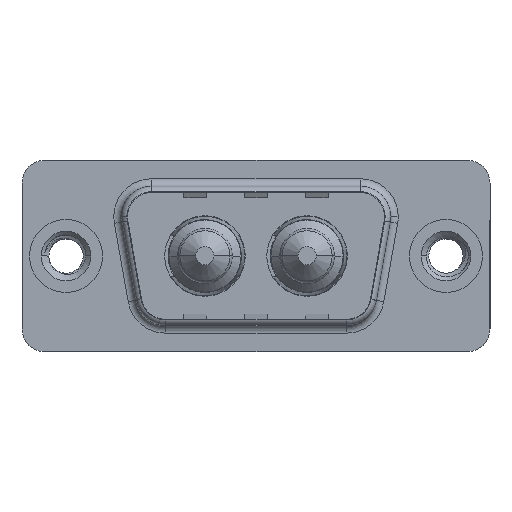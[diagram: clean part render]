
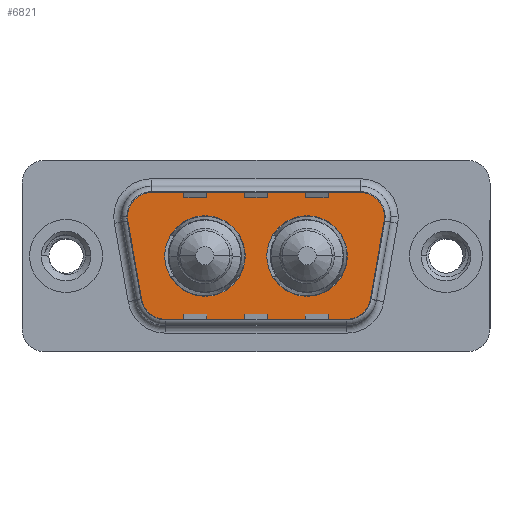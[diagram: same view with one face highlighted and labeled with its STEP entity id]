
A CAD part, top view. The second image highlights one B-rep face of the part: STEP entity #6821.
In plain terms, the highlighted planar face has unit normal (0, 0, 1).
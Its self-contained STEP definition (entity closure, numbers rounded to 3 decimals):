
#55 = DIRECTION ( 'NONE',  ( 1., 0., 0. ) ) ;
#293 = EDGE_CURVE ( 'NONE', #538, #6343, #3353, .T. ) ;
#428 = CARTESIAN_POINT ( 'NONE',  ( 5.436, 4.9, 0. ) ) ;
#538 = VERTEX_POINT ( 'NONE', #7679 ) ;
#563 = CARTESIAN_POINT ( 'NONE',  ( 19.564, 2.9, 0. ) ) ;
#599 = DIRECTION ( 'NONE',  ( 0., 0., 1. ) ) ;
#717 = CARTESIAN_POINT ( 'NONE',  ( 3.466, 2.553, 0. ) ) ;
#746 = AXIS2_PLACEMENT_3D ( 'NONE', #1592, #10124, #2827 ) ;
#830 = CARTESIAN_POINT ( 'NONE',  ( 6.49, 0., 0. ) ) ;
#866 = CARTESIAN_POINT ( 'NONE',  ( 21.534, 2.553, 0. ) ) ;
#883 = CIRCLE ( 'NONE', #5592, 2. ) ;
#1329 = AXIS2_PLACEMENT_3D ( 'NONE', #5317, #13799, #6526 ) ;
#1493 = VECTOR ( 'NONE', #1997, 1000. ) ;
#1539 = VERTEX_POINT ( 'NONE', #830 ) ;
#1551 = VERTEX_POINT ( 'NONE', #10765 ) ;
#1585 = CARTESIAN_POINT ( 'NONE',  ( 6.459, -4.9, 0. ) ) ;
#1592 = CARTESIAN_POINT ( 'NONE',  ( 15.86, 0., 0. ) ) ;
#1773 = DIRECTION ( 'NONE',  ( -1., 0., 0. ) ) ;
#1788 = DIRECTION ( 'NONE',  ( 1., 0., 0. ) ) ;
#1823 = CIRCLE ( 'NONE', #6727, 2. ) ;
#1856 = VERTEX_POINT ( 'NONE', #9873 ) ;
#1989 = DIRECTION ( 'NONE',  ( 0.174, -0.985, 0. ) ) ;
#1997 = DIRECTION ( 'NONE',  ( 0.174, 0.985, 0. ) ) ;
#2703 = DIRECTION ( 'NONE',  ( 0., 0., 1. ) ) ;
#2827 = DIRECTION ( 'NONE',  ( 1., 0., 0. ) ) ;
#2969 = VECTOR ( 'NONE', #1989, 1000. ) ;
#3025 = FACE_OUTER_BOUND ( 'NONE', #11076, .T. ) ;
#3049 = CIRCLE ( 'NONE', #9756, 2. ) ;
#3152 = CIRCLE ( 'NONE', #746, 2.65 ) ;
#3353 = LINE ( 'NONE', #4922, #12299 ) ;
#3422 = EDGE_CURVE ( 'NONE', #1551, #7633, #13109, .T. ) ;
#3642 = EDGE_LOOP ( 'NONE', ( #8192, #15733 ) ) ;
#3718 = CARTESIAN_POINT ( 'NONE',  ( 4.489, -3.247, 0. ) ) ;
#3866 = DIRECTION ( 'NONE',  ( 1., 0., 0. ) ) ;
#4012 = DIRECTION ( 'NONE',  ( 1., 0., 0. ) ) ;
#4110 = CARTESIAN_POINT ( 'NONE',  ( 19.564, 2.9, 0. ) ) ;
#4141 = VERTEX_POINT ( 'NONE', #13921 ) ;
#4147 = DIRECTION ( 'NONE',  ( -1., 0., 0. ) ) ;
#4219 = PLANE ( 'NONE',  #15092 ) ;
#4314 = EDGE_CURVE ( 'NONE', #1856, #4745, #14405, .T. ) ;
#4329 = VECTOR ( 'NONE', #7620, 1000. ) ;
#4400 = DIRECTION ( 'NONE',  ( 1., 0., 0. ) ) ;
#4431 = ORIENTED_EDGE ( 'NONE', *, *, #9809, .T. ) ;
#4470 = CARTESIAN_POINT ( 'NONE',  ( 21.534, 2.553, 0. ) ) ;
#4663 = DIRECTION ( 'NONE',  ( 0., 0., 1. ) ) ;
#4745 = VERTEX_POINT ( 'NONE', #866 ) ;
#4808 = VERTEX_POINT ( 'NONE', #3718 ) ;
#4902 = CIRCLE ( 'NONE', #13381, 2.65 ) ;
#4922 = CARTESIAN_POINT ( 'NONE',  ( 5.436, 4.9, 0. ) ) ;
#5101 = EDGE_CURVE ( 'NONE', #1539, #8948, #8860, .T. ) ;
#5166 = EDGE_CURVE ( 'NONE', #8948, #1539, #4902, .T. ) ;
#5316 = DIRECTION ( 'NONE',  ( -1., 0., 0. ) ) ;
#5317 = CARTESIAN_POINT ( 'NONE',  ( 6.459, -2.9, 0. ) ) ;
#5384 = AXIS2_PLACEMENT_3D ( 'NONE', #563, #9035, #1773 ) ;
#5399 = CARTESIAN_POINT ( 'NONE',  ( 18.541, -2.9, 0. ) ) ;
#5592 = AXIS2_PLACEMENT_3D ( 'NONE', #4110, #12606, #5316 ) ;
#5746 = VERTEX_POINT ( 'NONE', #7340 ) ;
#6104 = EDGE_CURVE ( 'NONE', #6343, #12043, #1823, .T. ) ;
#6165 = EDGE_LOOP ( 'NONE', ( #12387, #10317 ) ) ;
#6197 = LINE ( 'NONE', #717, #2969 ) ;
#6218 = CIRCLE ( 'NONE', #5384, 2. ) ;
#6321 = EDGE_CURVE ( 'NONE', #7633, #1551, #3152, .T. ) ;
#6343 = VERTEX_POINT ( 'NONE', #428 ) ;
#6526 = DIRECTION ( 'NONE',  ( -1., 0., 0. ) ) ;
#6613 = FACE_BOUND ( 'NONE', #3642, .T. ) ;
#6727 = AXIS2_PLACEMENT_3D ( 'NONE', #14624, #7315, #55 ) ;
#6821 = ADVANCED_FACE ( 'NONE', ( #13093, #6613, #3025 ), #4219, .T. ) ;
#6941 = CARTESIAN_POINT ( 'NONE',  ( 13.21, 0., 0. ) ) ;
#7241 = ORIENTED_EDGE ( 'NONE', *, *, #13550, .T. ) ;
#7315 = DIRECTION ( 'NONE',  ( 0., 0., 1. ) ) ;
#7340 = CARTESIAN_POINT ( 'NONE',  ( 18.541, -4.9, 0. ) ) ;
#7429 = CARTESIAN_POINT ( 'NONE',  ( 15.86, 0., 0. ) ) ;
#7620 = DIRECTION ( 'NONE',  ( 1., 0., 0. ) ) ;
#7633 = VERTEX_POINT ( 'NONE', #6941 ) ;
#7679 = CARTESIAN_POINT ( 'NONE',  ( 19.564, 4.9, 0. ) ) ;
#8192 = ORIENTED_EDGE ( 'NONE', *, *, #5166, .F. ) ;
#8565 = ORIENTED_EDGE ( 'NONE', *, *, #8621, .T. ) ;
#8621 = EDGE_CURVE ( 'NONE', #12043, #4808, #6197, .T. ) ;
#8741 = CARTESIAN_POINT ( 'NONE',  ( 9.14, 0., 0. ) ) ;
#8748 = AXIS2_PLACEMENT_3D ( 'NONE', #7429, #4663, #3866 ) ;
#8860 = CIRCLE ( 'NONE', #10159, 2.65 ) ;
#8948 = VERTEX_POINT ( 'NONE', #9760 ) ;
#9035 = DIRECTION ( 'NONE',  ( 0., 0., 1. ) ) ;
#9057 = DIRECTION ( 'NONE',  ( 0., 0., 1. ) ) ;
#9194 = EDGE_CURVE ( 'NONE', #4808, #14980, #14551, .T. ) ;
#9359 = ORIENTED_EDGE ( 'NONE', *, *, #12990, .T. ) ;
#9556 = ORIENTED_EDGE ( 'NONE', *, *, #293, .T. ) ;
#9738 = ORIENTED_EDGE ( 'NONE', *, *, #9194, .T. ) ;
#9756 = AXIS2_PLACEMENT_3D ( 'NONE', #9983, #2703, #11215 ) ;
#9760 = CARTESIAN_POINT ( 'NONE',  ( 11.79, 0., 0. ) ) ;
#9809 = EDGE_CURVE ( 'NONE', #14980, #5746, #13982, .T. ) ;
#9873 = CARTESIAN_POINT ( 'NONE',  ( 20.511, -3.247, 0. ) ) ;
#9983 = CARTESIAN_POINT ( 'NONE',  ( 18.541, -2.9, 0. ) ) ;
#10124 = DIRECTION ( 'NONE',  ( 0., 0., 1. ) ) ;
#10159 = AXIS2_PLACEMENT_3D ( 'NONE', #15430, #13688, #4012 ) ;
#10317 = ORIENTED_EDGE ( 'NONE', *, *, #6321, .F. ) ;
#10421 = ORIENTED_EDGE ( 'NONE', *, *, #11082, .T. ) ;
#10713 = ORIENTED_EDGE ( 'NONE', *, *, #6104, .T. ) ;
#10755 = CARTESIAN_POINT ( 'NONE',  ( 3.466, 2.553, 0. ) ) ;
#10765 = CARTESIAN_POINT ( 'NONE',  ( 18.51, 0., 0. ) ) ;
#11076 = EDGE_LOOP ( 'NONE', ( #10421, #11762, #9359, #7241, #9556, #10713, #8565, #9738, #4431 ) ) ;
#11082 = EDGE_CURVE ( 'NONE', #5746, #1856, #3049, .T. ) ;
#11215 = DIRECTION ( 'NONE',  ( 1., 0., 0. ) ) ;
#11762 = ORIENTED_EDGE ( 'NONE', *, *, #4314, .T. ) ;
#12043 = VERTEX_POINT ( 'NONE', #10755 ) ;
#12299 = VECTOR ( 'NONE', #4147, 1000. ) ;
#12387 = ORIENTED_EDGE ( 'NONE', *, *, #3422, .F. ) ;
#12606 = DIRECTION ( 'NONE',  ( 0., 0., 1. ) ) ;
#12990 = EDGE_CURVE ( 'NONE', #4745, #4141, #6218, .T. ) ;
#13093 = FACE_BOUND ( 'NONE', #6165, .T. ) ;
#13109 = CIRCLE ( 'NONE', #8748, 2.65 ) ;
#13381 = AXIS2_PLACEMENT_3D ( 'NONE', #8741, #599, #4400 ) ;
#13550 = EDGE_CURVE ( 'NONE', #4141, #538, #883, .T. ) ;
#13688 = DIRECTION ( 'NONE',  ( 0., 0., 1. ) ) ;
#13799 = DIRECTION ( 'NONE',  ( 0., 0., 1. ) ) ;
#13921 = CARTESIAN_POINT ( 'NONE',  ( 21.564, 2.9, 0. ) ) ;
#13982 = LINE ( 'NONE', #1585, #4329 ) ;
#14008 = CARTESIAN_POINT ( 'NONE',  ( 6.459, -4.9, 0. ) ) ;
#14405 = LINE ( 'NONE', #4470, #1493 ) ;
#14551 = CIRCLE ( 'NONE', #1329, 2. ) ;
#14624 = CARTESIAN_POINT ( 'NONE',  ( 5.436, 2.9, 0. ) ) ;
#14980 = VERTEX_POINT ( 'NONE', #14008 ) ;
#15092 = AXIS2_PLACEMENT_3D ( 'NONE', #5399, #9057, #1788 ) ;
#15430 = CARTESIAN_POINT ( 'NONE',  ( 9.14, 0., 0. ) ) ;
#15733 = ORIENTED_EDGE ( 'NONE', *, *, #5101, .F. ) ;
